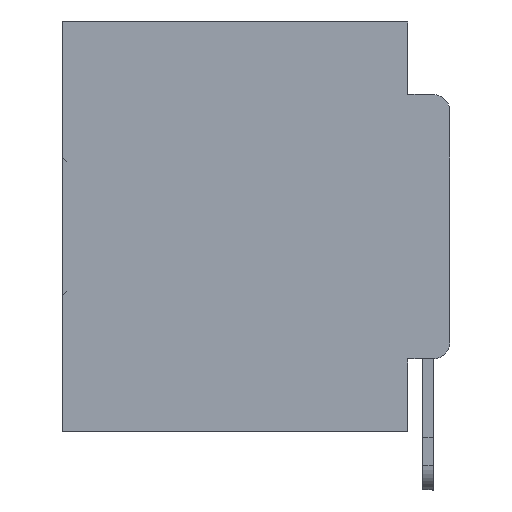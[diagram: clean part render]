
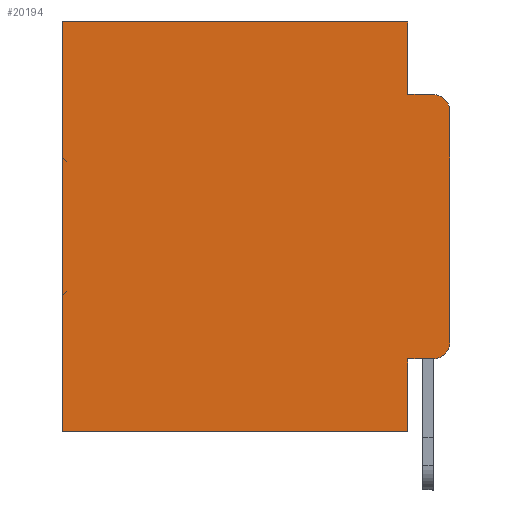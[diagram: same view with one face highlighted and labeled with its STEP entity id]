
A CAD part, left-side view. The second image highlights one B-rep face of the part: STEP entity #20194.
In plain terms, the highlighted planar face has unit normal (-1, 0, 0).
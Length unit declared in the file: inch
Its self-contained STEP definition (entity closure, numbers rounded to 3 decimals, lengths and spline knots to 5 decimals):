
#393 = DIRECTION ( 'NONE',  ( 0., 0., -1. ) ) ;
#418 = CARTESIAN_POINT ( 'NONE',  ( 0.298, 0.473, -0.5 ) ) ;
#484 = VECTOR ( 'NONE', #9987, 39.37008 ) ;
#896 = EDGE_CURVE ( 'NONE', #6785, #28527, #19790, .T. ) ;
#1546 = CARTESIAN_POINT ( 'NONE',  ( 0.298, 0.051, 0. ) ) ;
#1564 = CARTESIAN_POINT ( 'NONE',  ( 0.298, 0.051, -0.4115 ) ) ;
#2679 = PLANE ( 'NONE',  #25872 ) ;
#3460 = CARTESIAN_POINT ( 'NONE',  ( 0.298, 0.051, -0.0885 ) ) ;
#3554 = EDGE_LOOP ( 'NONE', ( #12485, #16048, #32675, #22620, #16165, #7487, #27517, #29788, #12488, #8779 ) ) ;
#4776 = AXIS2_PLACEMENT_3D ( 'NONE', #10190, #7598, #15950 ) ;
#4910 = CARTESIAN_POINT ( 'NONE',  ( 0.298, 0.051, -0.5 ) ) ;
#6578 = CARTESIAN_POINT ( 'NONE',  ( 0.298, 0.051, -0.4115 ) ) ;
#6785 = VERTEX_POINT ( 'NONE', #17543 ) ;
#7018 = VECTOR ( 'NONE', #16607, 39.37008 ) ;
#7487 = ORIENTED_EDGE ( 'NONE', *, *, #24539, .T. ) ;
#7598 = DIRECTION ( 'NONE',  ( -1., 0., 0. ) ) ;
#7732 = CARTESIAN_POINT ( 'NONE',  ( 0.298, 0.051, -0.0885 ) ) ;
#8779 = ORIENTED_EDGE ( 'NONE', *, *, #896, .T. ) ;
#9624 = CARTESIAN_POINT ( 'NONE',  ( 0.298, 0., -0.5 ) ) ;
#9973 = DIRECTION ( 'NONE',  ( 0., 0., -1. ) ) ;
#9987 = DIRECTION ( 'NONE',  ( 0., 0., -1. ) ) ;
#10190 = CARTESIAN_POINT ( 'NONE',  ( 0.298, 0.02, -0.3915 ) ) ;
#10341 = VECTOR ( 'NONE', #29707, 39.37008 ) ;
#11012 = VECTOR ( 'NONE', #14094, 39.37008 ) ;
#11030 = DIRECTION ( 'NONE',  ( 0., 1., 0. ) ) ;
#11192 = CARTESIAN_POINT ( 'NONE',  ( 0.298, 0.051, 0. ) ) ;
#11729 = DIRECTION ( 'NONE',  ( 0., 0., -1. ) ) ;
#12170 = VECTOR ( 'NONE', #11729, 39.37008 ) ;
#12251 = LINE ( 'NONE', #30760, #12170 ) ;
#12485 = ORIENTED_EDGE ( 'NONE', *, *, #27302, .F. ) ;
#12488 = ORIENTED_EDGE ( 'NONE', *, *, #14805, .T. ) ;
#12750 = LINE ( 'NONE', #9624, #31025 ) ;
#12889 = CARTESIAN_POINT ( 'NONE',  ( 0.298, 0.473, 0. ) ) ;
#12920 = CARTESIAN_POINT ( 'NONE',  ( 0.298, 0.02, -0.1085 ) ) ;
#13117 = LINE ( 'NONE', #26049, #484 ) ;
#13173 = VERTEX_POINT ( 'NONE', #26678 ) ;
#13472 = CARTESIAN_POINT ( 'NONE',  ( 0.298, 0.473, 0. ) ) ;
#13992 = CARTESIAN_POINT ( 'NONE',  ( 0.298, 0., 0. ) ) ;
#14094 = DIRECTION ( 'NONE',  ( 0., -1., 0. ) ) ;
#14435 = CIRCLE ( 'NONE', #16652, 0.02 ) ;
#14805 = EDGE_CURVE ( 'NONE', #22540, #6785, #17778, .T. ) ;
#15950 = DIRECTION ( 'NONE',  ( 0., 0., -1. ) ) ;
#16048 = ORIENTED_EDGE ( 'NONE', *, *, #20491, .T. ) ;
#16165 = ORIENTED_EDGE ( 'NONE', *, *, #17208, .T. ) ;
#16607 = DIRECTION ( 'NONE',  ( 0., 0., -1. ) ) ;
#16652 = AXIS2_PLACEMENT_3D ( 'NONE', #12920, #33724, #9973 ) ;
#16853 = VECTOR ( 'NONE', #11030, 39.37008 ) ;
#17208 = EDGE_CURVE ( 'NONE', #28220, #26607, #26915, .T. ) ;
#17543 = CARTESIAN_POINT ( 'NONE',  ( 0.298, 0.02, -0.4115 ) ) ;
#17778 = LINE ( 'NONE', #1564, #31374 ) ;
#19236 = EDGE_CURVE ( 'NONE', #23461, #25623, #12750, .T. ) ;
#19497 = LINE ( 'NONE', #3460, #11012 ) ;
#19790 = CIRCLE ( 'NONE', #4776, 0.02 ) ;
#20194 = ADVANCED_FACE ( 'NONE', ( #29712 ), #2679, .F. ) ;
#20491 = EDGE_CURVE ( 'NONE', #13173, #26979, #14435, .T. ) ;
#21738 = CARTESIAN_POINT ( 'NONE',  ( 0.298, 0., -0.3915 ) ) ;
#22540 = VERTEX_POINT ( 'NONE', #6578 ) ;
#22620 = ORIENTED_EDGE ( 'NONE', *, *, #24541, .F. ) ;
#22647 = CARTESIAN_POINT ( 'NONE',  ( 0.298, 0.02, -0.0885 ) ) ;
#23461 = VERTEX_POINT ( 'NONE', #4910 ) ;
#24107 = LINE ( 'NONE', #11192, #7018 ) ;
#24539 = EDGE_CURVE ( 'NONE', #26607, #25623, #32155, .T. ) ;
#24541 = EDGE_CURVE ( 'NONE', #28220, #31829, #24107, .T. ) ;
#25623 = VERTEX_POINT ( 'NONE', #418 ) ;
#25805 = DIRECTION ( 'NONE',  ( 0., -1., 0. ) ) ;
#25872 = AXIS2_PLACEMENT_3D ( 'NONE', #34435, #29021, #393 ) ;
#26049 = CARTESIAN_POINT ( 'NONE',  ( 0.298, 0.051, 0. ) ) ;
#26607 = VERTEX_POINT ( 'NONE', #12889 ) ;
#26678 = CARTESIAN_POINT ( 'NONE',  ( 0.298, 0., -0.1085 ) ) ;
#26915 = LINE ( 'NONE', #13992, #16853 ) ;
#26979 = VERTEX_POINT ( 'NONE', #22647 ) ;
#27302 = EDGE_CURVE ( 'NONE', #13173, #28527, #12251, .T. ) ;
#27322 = EDGE_CURVE ( 'NONE', #22540, #23461, #13117, .T. ) ;
#27517 = ORIENTED_EDGE ( 'NONE', *, *, #19236, .F. ) ;
#28172 = EDGE_CURVE ( 'NONE', #31829, #26979, #19497, .T. ) ;
#28220 = VERTEX_POINT ( 'NONE', #1546 ) ;
#28294 = DIRECTION ( 'NONE',  ( 0., 1., 0. ) ) ;
#28527 = VERTEX_POINT ( 'NONE', #21738 ) ;
#29021 = DIRECTION ( 'NONE',  ( 1., 0., 0. ) ) ;
#29707 = DIRECTION ( 'NONE',  ( 0., 0., -1. ) ) ;
#29712 = FACE_OUTER_BOUND ( 'NONE', #3554, .T. ) ;
#29788 = ORIENTED_EDGE ( 'NONE', *, *, #27322, .F. ) ;
#30760 = CARTESIAN_POINT ( 'NONE',  ( 0.298, 0., 0. ) ) ;
#31025 = VECTOR ( 'NONE', #28294, 39.37008 ) ;
#31374 = VECTOR ( 'NONE', #25805, 39.37008 ) ;
#31829 = VERTEX_POINT ( 'NONE', #7732 ) ;
#32155 = LINE ( 'NONE', #13472, #10341 ) ;
#32675 = ORIENTED_EDGE ( 'NONE', *, *, #28172, .F. ) ;
#33724 = DIRECTION ( 'NONE',  ( -1., 0., 0. ) ) ;
#34435 = CARTESIAN_POINT ( 'NONE',  ( 0.298, 0., 0. ) ) ;
